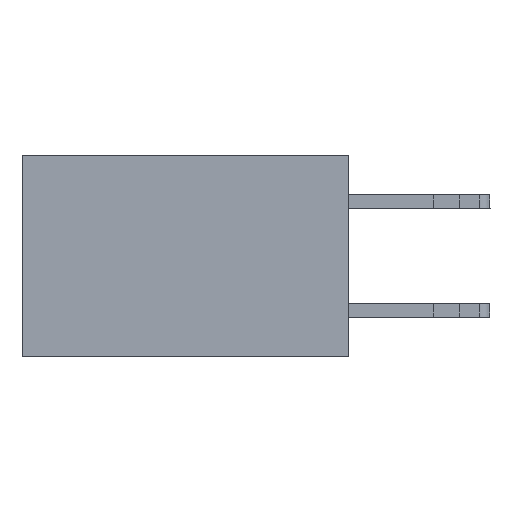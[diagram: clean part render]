
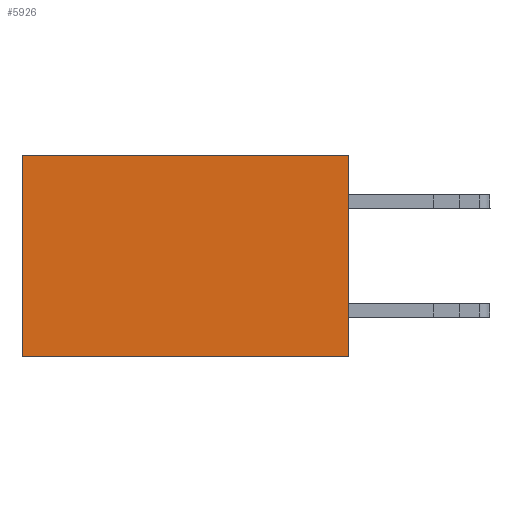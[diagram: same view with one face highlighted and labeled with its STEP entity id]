
A CAD part, left-side view. The second image highlights one B-rep face of the part: STEP entity #5926.
In plain terms, the highlighted planar face has unit normal (-1, 0, 0).
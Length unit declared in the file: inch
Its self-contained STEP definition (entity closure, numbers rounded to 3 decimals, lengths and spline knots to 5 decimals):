
#772 = VERTEX_POINT ( 'NONE', #16698 ) ;
#1277 = AXIS2_PLACEMENT_3D ( 'NONE', #11236, #9786, #2487 ) ;
#2487 = DIRECTION ( 'NONE',  ( 0., 0., -1. ) ) ;
#4116 = VECTOR ( 'NONE', #11533, 39.37008 ) ;
#4266 = DIRECTION ( 'NONE',  ( 0., 0., -1. ) ) ;
#4437 = DIRECTION ( 'NONE',  ( 0., 0., -1. ) ) ;
#4545 = DIRECTION ( 'NONE',  ( 0., 1., 0. ) ) ;
#5282 = PLANE ( 'NONE',  #1277 ) ;
#5900 = LINE ( 'NONE', #13097, #18869 ) ;
#5920 = LINE ( 'NONE', #18807, #18912 ) ;
#5926 = ADVANCED_FACE ( 'NONE', ( #6723 ), #5282, .F. ) ;
#5997 = VERTEX_POINT ( 'NONE', #10439 ) ;
#6723 = FACE_OUTER_BOUND ( 'NONE', #13337, .T. ) ;
#6780 = ORIENTED_EDGE ( 'NONE', *, *, #9462, .F. ) ;
#7992 = CARTESIAN_POINT ( 'NONE',  ( 0.2615, 0.6, 0. ) ) ;
#9084 = VECTOR ( 'NONE', #4437, 39.37008 ) ;
#9106 = EDGE_CURVE ( 'NONE', #13506, #16322, #5920, .T. ) ;
#9462 = EDGE_CURVE ( 'NONE', #5997, #772, #16184, .T. ) ;
#9786 = DIRECTION ( 'NONE',  ( 1., 0., 0. ) ) ;
#10439 = CARTESIAN_POINT ( 'NONE',  ( 0.2615, 0., 0. ) ) ;
#10907 = EDGE_CURVE ( 'NONE', #772, #16322, #5900, .T. ) ;
#11236 = CARTESIAN_POINT ( 'NONE',  ( 0.2615, 0., -0.37 ) ) ;
#11437 = EDGE_CURVE ( 'NONE', #5997, #13506, #14435, .T. ) ;
#11533 = DIRECTION ( 'NONE',  ( 0., 1., 0. ) ) ;
#11643 = CARTESIAN_POINT ( 'NONE',  ( 0.2615, 0., -0.37 ) ) ;
#12980 = CARTESIAN_POINT ( 'NONE',  ( 0.2615, 0., 0. ) ) ;
#13097 = CARTESIAN_POINT ( 'NONE',  ( 0.2615, 0., -0.37 ) ) ;
#13337 = EDGE_LOOP ( 'NONE', ( #14793, #16199, #6780, #18484 ) ) ;
#13506 = VERTEX_POINT ( 'NONE', #7992 ) ;
#14435 = LINE ( 'NONE', #12980, #4116 ) ;
#14793 = ORIENTED_EDGE ( 'NONE', *, *, #9106, .T. ) ;
#16184 = LINE ( 'NONE', #11643, #9084 ) ;
#16199 = ORIENTED_EDGE ( 'NONE', *, *, #10907, .F. ) ;
#16322 = VERTEX_POINT ( 'NONE', #16543 ) ;
#16543 = CARTESIAN_POINT ( 'NONE',  ( 0.2615, 0.6, -0.37 ) ) ;
#16698 = CARTESIAN_POINT ( 'NONE',  ( 0.2615, 0., -0.37 ) ) ;
#18484 = ORIENTED_EDGE ( 'NONE', *, *, #11437, .T. ) ;
#18807 = CARTESIAN_POINT ( 'NONE',  ( 0.2615, 0.6, -0.37 ) ) ;
#18869 = VECTOR ( 'NONE', #4545, 39.37008 ) ;
#18912 = VECTOR ( 'NONE', #4266, 39.37008 ) ;
